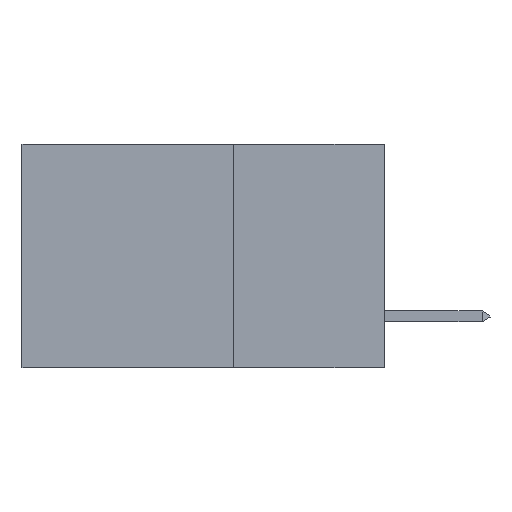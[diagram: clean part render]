
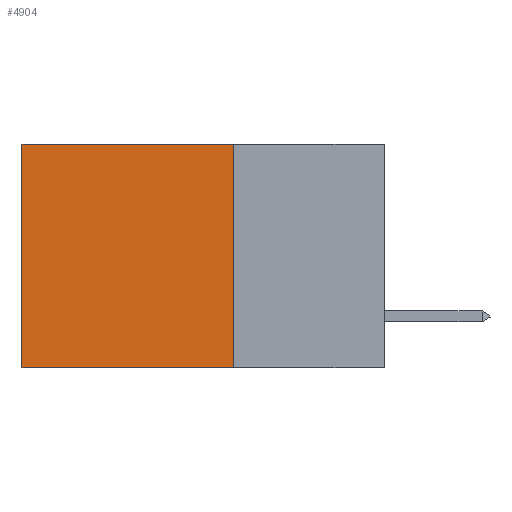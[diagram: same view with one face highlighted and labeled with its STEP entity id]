
A CAD part, left-side view. The second image highlights one B-rep face of the part: STEP entity #4904.
In plain terms, the highlighted planar face has unit normal (-1, 0, 0).
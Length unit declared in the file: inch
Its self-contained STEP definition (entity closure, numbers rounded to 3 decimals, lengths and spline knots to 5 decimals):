
#477 = CARTESIAN_POINT ( 'NONE',  ( 0.2875, 0.6, 0. ) ) ;
#605 = ORIENTED_EDGE ( 'NONE', *, *, #3656, .T. ) ;
#887 = VECTOR ( 'NONE', #1532, 39.37008 ) ;
#932 = ORIENTED_EDGE ( 'NONE', *, *, #5135, .T. ) ;
#940 = CARTESIAN_POINT ( 'NONE',  ( 0.2875, 0.25, -0.37 ) ) ;
#1361 = CARTESIAN_POINT ( 'NONE',  ( 0.2875, 0.6, -0.37 ) ) ;
#1419 = ORIENTED_EDGE ( 'NONE', *, *, #12537, .F. ) ;
#1532 = DIRECTION ( 'NONE',  ( 0., 1., 0. ) ) ;
#1600 = LINE ( 'NONE', #1728, #13373 ) ;
#1728 = CARTESIAN_POINT ( 'NONE',  ( 0.2875, 0.6, 0. ) ) ;
#1888 = AXIS2_PLACEMENT_3D ( 'NONE', #4405, #4451, #7592 ) ;
#2130 = CARTESIAN_POINT ( 'NONE',  ( 0.2875, 0.25, 0. ) ) ;
#2165 = DIRECTION ( 'NONE',  ( 0., 0., -1. ) ) ;
#3355 = VERTEX_POINT ( 'NONE', #1361 ) ;
#3556 = LINE ( 'NONE', #7959, #887 ) ;
#3656 = EDGE_CURVE ( 'NONE', #10937, #3355, #1600, .T. ) ;
#4330 = LINE ( 'NONE', #7770, #9297 ) ;
#4405 = CARTESIAN_POINT ( 'NONE',  ( 0.2875, 0.25, 0. ) ) ;
#4451 = DIRECTION ( 'NONE',  ( 1., 0., 0. ) ) ;
#4904 = ADVANCED_FACE ( 'NONE', ( #9366 ), #9926, .F. ) ;
#5135 = EDGE_CURVE ( 'NONE', #8115, #10937, #3556, .T. ) ;
#6061 = DIRECTION ( 'NONE',  ( 0., 0., -1. ) ) ;
#7491 = VERTEX_POINT ( 'NONE', #940 ) ;
#7592 = DIRECTION ( 'NONE',  ( 0., 0., -1. ) ) ;
#7764 = EDGE_LOOP ( 'NONE', ( #605, #1419, #8876, #932 ) ) ;
#7770 = CARTESIAN_POINT ( 'NONE',  ( 0.2875, 0.25, -0.37 ) ) ;
#7819 = DIRECTION ( 'NONE',  ( 0., 1., 0. ) ) ;
#7959 = CARTESIAN_POINT ( 'NONE',  ( 0.2875, 0.25, 0. ) ) ;
#8115 = VERTEX_POINT ( 'NONE', #2130 ) ;
#8392 = LINE ( 'NONE', #12749, #9715 ) ;
#8876 = ORIENTED_EDGE ( 'NONE', *, *, #9100, .F. ) ;
#9100 = EDGE_CURVE ( 'NONE', #8115, #7491, #8392, .T. ) ;
#9297 = VECTOR ( 'NONE', #7819, 39.37008 ) ;
#9366 = FACE_OUTER_BOUND ( 'NONE', #7764, .T. ) ;
#9715 = VECTOR ( 'NONE', #2165, 39.37008 ) ;
#9926 = PLANE ( 'NONE',  #1888 ) ;
#10937 = VERTEX_POINT ( 'NONE', #477 ) ;
#12537 = EDGE_CURVE ( 'NONE', #7491, #3355, #4330, .T. ) ;
#12749 = CARTESIAN_POINT ( 'NONE',  ( 0.2875, 0.25, 0. ) ) ;
#13373 = VECTOR ( 'NONE', #6061, 39.37008 ) ;
